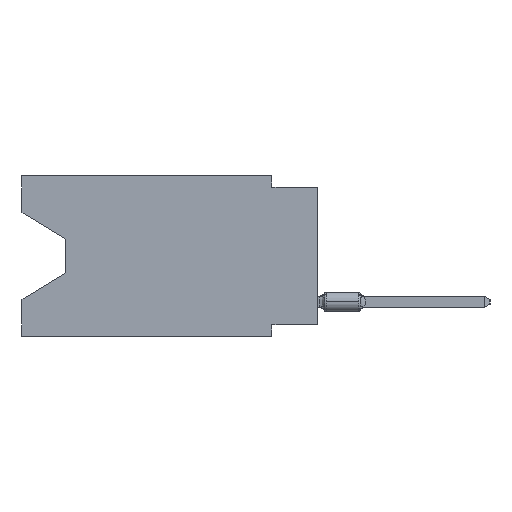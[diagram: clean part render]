
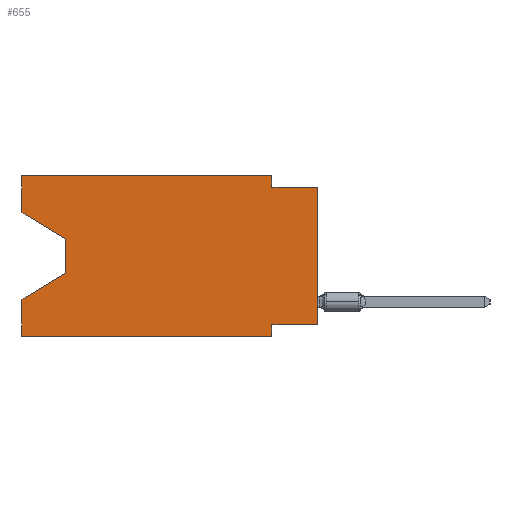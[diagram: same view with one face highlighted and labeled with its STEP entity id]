
A CAD part, left-side view. The second image highlights one B-rep face of the part: STEP entity #655.
In plain terms, the highlighted planar face has unit normal (-1, 0, 0).
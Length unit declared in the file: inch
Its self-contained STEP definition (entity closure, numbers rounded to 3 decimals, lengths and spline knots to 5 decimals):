
#655 = ADVANCED_FACE ( 'NONE', ( #2520 ), #11703, .F. ) ;
#1256 = VERTEX_POINT ( 'NONE', #9549 ) ;
#1290 = ORIENTED_EDGE ( 'NONE', *, *, #9361, .T. ) ;
#1545 = VERTEX_POINT ( 'NONE', #26925 ) ;
#1880 = CARTESIAN_POINT ( 'NONE',  ( 0., 0.645, -0.26975 ) ) ;
#2520 = FACE_OUTER_BOUND ( 'NONE', #7393, .T. ) ;
#2895 = LINE ( 'NONE', #15536, #50229 ) ;
#2978 = CARTESIAN_POINT ( 'NONE',  ( 0., 0.645, 0. ) ) ;
#3306 = EDGE_CURVE ( 'NONE', #6790, #49405, #37471, .T. ) ;
#3437 = CARTESIAN_POINT ( 'NONE',  ( 0., 0.645, -0.35 ) ) ;
#4945 = CARTESIAN_POINT ( 'NONE',  ( 0., 0., 0. ) ) ;
#5226 = CARTESIAN_POINT ( 'NONE',  ( 0., 0.55, -0.212 ) ) ;
#5591 = CARTESIAN_POINT ( 'NONE',  ( 0., 0.55, -0.138 ) ) ;
#6077 = DIRECTION ( 'NONE',  ( 0., 0., 1. ) ) ;
#6602 = CARTESIAN_POINT ( 'NONE',  ( 0., 0.645, 0. ) ) ;
#6752 = CARTESIAN_POINT ( 'NONE',  ( 0., 0., -0.325 ) ) ;
#6790 = VERTEX_POINT ( 'NONE', #31761 ) ;
#6853 = VECTOR ( 'NONE', #41795, 39.37008 ) ;
#7393 = EDGE_LOOP ( 'NONE', ( #12241, #27241, #48318, #19079, #40708, #36712, #48751, #1290, #28497, #38867, #29501, #7974 ) ) ;
#7974 = ORIENTED_EDGE ( 'NONE', *, *, #50017, .F. ) ;
#8372 = VECTOR ( 'NONE', #52164, 39.37008 ) ;
#9197 = LINE ( 'NONE', #26716, #12840 ) ;
#9361 = EDGE_CURVE ( 'NONE', #39431, #1256, #40837, .T. ) ;
#9391 = VERTEX_POINT ( 'NONE', #27602 ) ;
#9549 = CARTESIAN_POINT ( 'NONE',  ( 0., 0., -0.025 ) ) ;
#9898 = VECTOR ( 'NONE', #6077, 39.37008 ) ;
#10543 = EDGE_CURVE ( 'NONE', #1545, #43641, #53765, .T. ) ;
#11111 = DIRECTION ( 'NONE',  ( 0., 0.855, -0.519 ) ) ;
#11505 = DIRECTION ( 'NONE',  ( 0., 0., -1. ) ) ;
#11703 = PLANE ( 'NONE',  #16115 ) ;
#12217 = LINE ( 'NONE', #6752, #16514 ) ;
#12241 = ORIENTED_EDGE ( 'NONE', *, *, #17136, .T. ) ;
#12271 = EDGE_CURVE ( 'NONE', #53406, #24209, #2895, .T. ) ;
#12829 = CARTESIAN_POINT ( 'NONE',  ( 0., 0.645, -0.35 ) ) ;
#12840 = VECTOR ( 'NONE', #31321, 39.37008 ) ;
#14208 = LINE ( 'NONE', #31730, #38449 ) ;
#14409 = DIRECTION ( 'NONE',  ( 0., -1., 0. ) ) ;
#14935 = CARTESIAN_POINT ( 'NONE',  ( 0., 0.1, -0.025 ) ) ;
#15500 = LINE ( 'NONE', #6602, #25409 ) ;
#15513 = LINE ( 'NONE', #3437, #53165 ) ;
#15536 = CARTESIAN_POINT ( 'NONE',  ( 0., 0.55, -0.138 ) ) ;
#15611 = DIRECTION ( 'NONE',  ( 0., 0., 1. ) ) ;
#16115 = AXIS2_PLACEMENT_3D ( 'NONE', #20046, #32427, #49935 ) ;
#16514 = VECTOR ( 'NONE', #24278, 39.37008 ) ;
#16864 = EDGE_CURVE ( 'NONE', #24209, #49398, #36119, .T. ) ;
#17136 = EDGE_CURVE ( 'NONE', #9391, #53406, #42990, .T. ) ;
#19079 = ORIENTED_EDGE ( 'NONE', *, *, #24028, .F. ) ;
#20046 = CARTESIAN_POINT ( 'NONE',  ( 0., 0.645, 0. ) ) ;
#21221 = DIRECTION ( 'NONE',  ( 0., -1., 0. ) ) ;
#21255 = VECTOR ( 'NONE', #11111, 39.37008 ) ;
#23091 = EDGE_CURVE ( 'NONE', #40941, #1256, #14208, .T. ) ;
#24028 = EDGE_CURVE ( 'NONE', #45201, #49398, #15500, .T. ) ;
#24209 = VERTEX_POINT ( 'NONE', #5226 ) ;
#24278 = DIRECTION ( 'NONE',  ( 0., 1., 0. ) ) ;
#25409 = VECTOR ( 'NONE', #41655, 39.37008 ) ;
#26716 = CARTESIAN_POINT ( 'NONE',  ( 0., 0.1, 0. ) ) ;
#26925 = CARTESIAN_POINT ( 'NONE',  ( 0., 0.645, 0. ) ) ;
#26934 = CARTESIAN_POINT ( 'NONE',  ( 0., 0., -0.325 ) ) ;
#27241 = ORIENTED_EDGE ( 'NONE', *, *, #12271, .T. ) ;
#27602 = CARTESIAN_POINT ( 'NONE',  ( 0., 0.645, -0.08025 ) ) ;
#28102 = EDGE_CURVE ( 'NONE', #39431, #6790, #12217, .T. ) ;
#28497 = ORIENTED_EDGE ( 'NONE', *, *, #23091, .F. ) ;
#28579 = CARTESIAN_POINT ( 'NONE',  ( 0., 0.1, -0.35 ) ) ;
#29300 = DIRECTION ( 'NONE',  ( 0., -1., 0. ) ) ;
#29501 = ORIENTED_EDGE ( 'NONE', *, *, #10543, .F. ) ;
#31321 = DIRECTION ( 'NONE',  ( 0., 0., -1. ) ) ;
#31730 = CARTESIAN_POINT ( 'NONE',  ( 0., 0., -0.025 ) ) ;
#31761 = CARTESIAN_POINT ( 'NONE',  ( 0., 0.1, -0.325 ) ) ;
#32427 = DIRECTION ( 'NONE',  ( 1., 0., 0. ) ) ;
#36082 = CARTESIAN_POINT ( 'NONE',  ( 0., 0.1, -0.35 ) ) ;
#36119 = LINE ( 'NONE', #53631, #21255 ) ;
#36605 = VECTOR ( 'NONE', #15611, 39.37008 ) ;
#36712 = ORIENTED_EDGE ( 'NONE', *, *, #3306, .F. ) ;
#37471 = LINE ( 'NONE', #28579, #6853 ) ;
#38016 = LINE ( 'NONE', #2978, #36605 ) ;
#38449 = VECTOR ( 'NONE', #21221, 39.37008 ) ;
#38867 = ORIENTED_EDGE ( 'NONE', *, *, #41817, .F. ) ;
#39431 = VERTEX_POINT ( 'NONE', #26934 ) ;
#40708 = ORIENTED_EDGE ( 'NONE', *, *, #43320, .T. ) ;
#40837 = LINE ( 'NONE', #4945, #9898 ) ;
#40941 = VERTEX_POINT ( 'NONE', #14935 ) ;
#41655 = DIRECTION ( 'NONE',  ( 0., 0., 1. ) ) ;
#41795 = DIRECTION ( 'NONE',  ( 0., 0., -1. ) ) ;
#41817 = EDGE_CURVE ( 'NONE', #43641, #40941, #9197, .T. ) ;
#42990 = LINE ( 'NONE', #56220, #8372 ) ;
#43320 = EDGE_CURVE ( 'NONE', #45201, #49405, #15513, .T. ) ;
#43641 = VERTEX_POINT ( 'NONE', #44449 ) ;
#44449 = CARTESIAN_POINT ( 'NONE',  ( 0., 0.1, 0. ) ) ;
#45201 = VERTEX_POINT ( 'NONE', #12829 ) ;
#45642 = VECTOR ( 'NONE', #14409, 39.37008 ) ;
#48318 = ORIENTED_EDGE ( 'NONE', *, *, #16864, .T. ) ;
#48751 = ORIENTED_EDGE ( 'NONE', *, *, #28102, .F. ) ;
#49398 = VERTEX_POINT ( 'NONE', #1880 ) ;
#49405 = VERTEX_POINT ( 'NONE', #36082 ) ;
#49935 = DIRECTION ( 'NONE',  ( 0., 0., -1. ) ) ;
#50017 = EDGE_CURVE ( 'NONE', #9391, #1545, #38016, .T. ) ;
#50229 = VECTOR ( 'NONE', #11505, 39.37008 ) ;
#52164 = DIRECTION ( 'NONE',  ( 0., -0.855, -0.519 ) ) ;
#53165 = VECTOR ( 'NONE', #29300, 39.37008 ) ;
#53187 = CARTESIAN_POINT ( 'NONE',  ( 0., 0.645, 0. ) ) ;
#53406 = VERTEX_POINT ( 'NONE', #5591 ) ;
#53631 = CARTESIAN_POINT ( 'NONE',  ( 0., 0.55, -0.212 ) ) ;
#53765 = LINE ( 'NONE', #53187, #45642 ) ;
#56220 = CARTESIAN_POINT ( 'NONE',  ( 0., 0.645, -0.08025 ) ) ;
